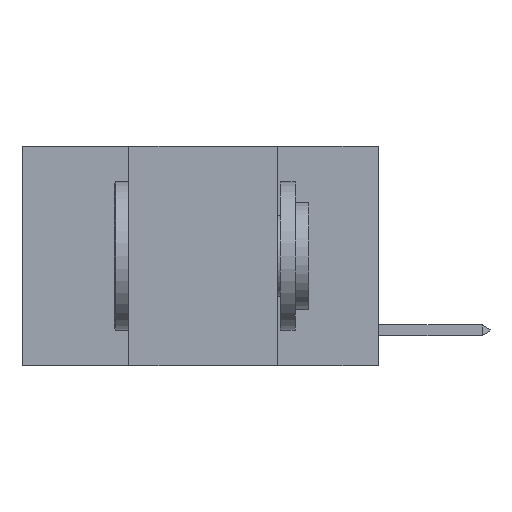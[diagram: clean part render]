
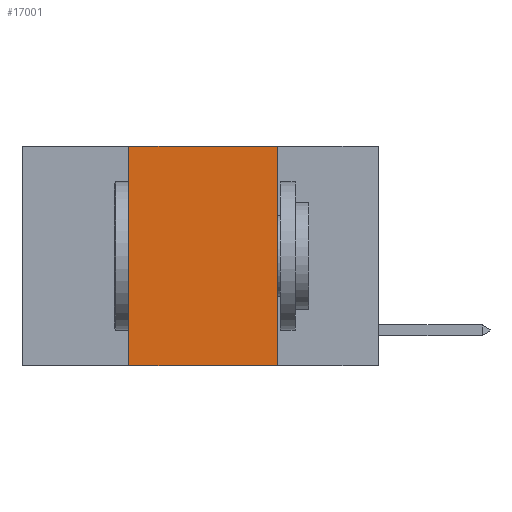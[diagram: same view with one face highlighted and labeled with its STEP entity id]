
A CAD part, left-side view. The second image highlights one B-rep face of the part: STEP entity #17001.
In plain terms, the highlighted planar face has unit normal (-1, 0, 0).
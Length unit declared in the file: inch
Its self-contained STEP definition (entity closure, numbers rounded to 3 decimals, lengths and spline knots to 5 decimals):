
#190 = PLANE ( 'NONE',  #26645 ) ;
#452 = VERTEX_POINT ( 'NONE', #1637 ) ;
#1204 = LINE ( 'NONE', #19901, #22458 ) ;
#1276 = VECTOR ( 'NONE', #12034, 39.37008 ) ;
#1314 = EDGE_CURVE ( 'NONE', #21289, #2078, #8756, .T. ) ;
#1637 = CARTESIAN_POINT ( 'NONE',  ( 0., 0.42, -0.37 ) ) ;
#2078 = VERTEX_POINT ( 'NONE', #25461 ) ;
#2337 = DIRECTION ( 'NONE',  ( 0., 0., -1. ) ) ;
#4360 = CARTESIAN_POINT ( 'NONE',  ( 0., 0.6, 0. ) ) ;
#4500 = LINE ( 'NONE', #16183, #15217 ) ;
#5109 = ORIENTED_EDGE ( 'NONE', *, *, #17183, .F. ) ;
#5780 = ORIENTED_EDGE ( 'NONE', *, *, #8006, .T. ) ;
#6992 = EDGE_LOOP ( 'NONE', ( #10134, #21411, #5109, #5780 ) ) ;
#8006 = EDGE_CURVE ( 'NONE', #452, #2078, #4500, .T. ) ;
#8756 = LINE ( 'NONE', #20783, #24340 ) ;
#9868 = CARTESIAN_POINT ( 'NONE',  ( 0., 0.6, 0. ) ) ;
#10134 = ORIENTED_EDGE ( 'NONE', *, *, #1314, .F. ) ;
#11726 = CARTESIAN_POINT ( 'NONE',  ( 0., 0.42, 0. ) ) ;
#12034 = DIRECTION ( 'NONE',  ( 0., -1., 0. ) ) ;
#12662 = LINE ( 'NONE', #9868, #1276 ) ;
#15128 = DIRECTION ( 'NONE',  ( 1., 0., 0. ) ) ;
#15217 = VECTOR ( 'NONE', #18322, 39.37008 ) ;
#15416 = EDGE_CURVE ( 'NONE', #20234, #21289, #12662, .T. ) ;
#16183 = CARTESIAN_POINT ( 'NONE',  ( 0., 0.6, -0.37 ) ) ;
#16580 = FACE_OUTER_BOUND ( 'NONE', #6992, .T. ) ;
#17001 = ADVANCED_FACE ( 'NONE', ( #16580 ), #190, .F. ) ;
#17183 = EDGE_CURVE ( 'NONE', #452, #20234, #1204, .T. ) ;
#17347 = CARTESIAN_POINT ( 'NONE',  ( 0., 0.17, 0. ) ) ;
#18322 = DIRECTION ( 'NONE',  ( 0., -1., 0. ) ) ;
#19901 = CARTESIAN_POINT ( 'NONE',  ( 0., 0.42, 0. ) ) ;
#20142 = DIRECTION ( 'NONE',  ( 0., 0., -1. ) ) ;
#20234 = VERTEX_POINT ( 'NONE', #11726 ) ;
#20783 = CARTESIAN_POINT ( 'NONE',  ( 0., 0.17, 0. ) ) ;
#21289 = VERTEX_POINT ( 'NONE', #17347 ) ;
#21411 = ORIENTED_EDGE ( 'NONE', *, *, #15416, .F. ) ;
#22458 = VECTOR ( 'NONE', #26216, 39.37008 ) ;
#24340 = VECTOR ( 'NONE', #20142, 39.37008 ) ;
#25461 = CARTESIAN_POINT ( 'NONE',  ( 0., 0.17, -0.37 ) ) ;
#26216 = DIRECTION ( 'NONE',  ( 0., 0., 1. ) ) ;
#26645 = AXIS2_PLACEMENT_3D ( 'NONE', #4360, #15128, #2337 ) ;
